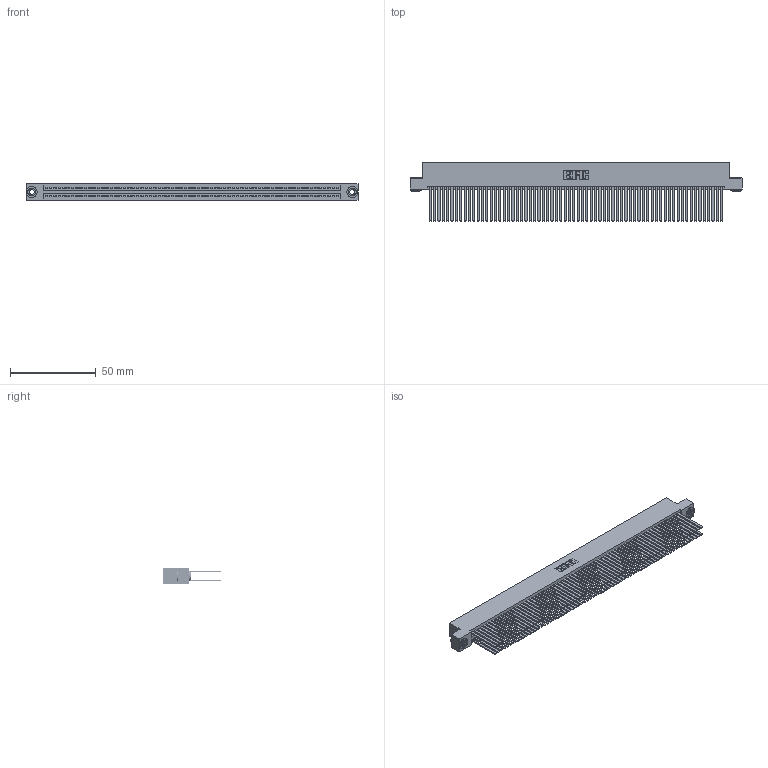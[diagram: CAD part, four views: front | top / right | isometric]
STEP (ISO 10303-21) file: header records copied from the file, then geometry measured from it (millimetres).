
FILE_DESCRIPTION (( 'STEP AP203' ), '1' );
FILE_NAME ('345-136-544-203.STEP', '2019-11-08T09:29:39', ( '' ), ( '' ), 'SwSTEP 2.0', 'SolidWorks 2016', '' );
FILE_SCHEMA (( 'CONFIG_CONTROL_DESIGN' ));
Length unit declared in the file: inch
Products named in the file (4): 345-250-002_345-250-002-102; 345-292-001_345-293-144; 345 Part_Flush Mounting Lugs - 0.156 Dia-TH; 345-136-544-203
Assembly tree (139 placements, depth 2):
  345-136-544-203
    345 Part_Flush Mounting Lugs - 0.156 Dia-TH
    345-292-001_345-293-144  x136
    345-250-002_345-250-002-102  x2
Bounding box: 193.93 x 33.96 x 9.4 mm (x, y, z)
Volume: 21005.7 mm3; surface area: 37346.1 mm2
Topology: 139 solids, 139 shells, 6148 faces, 18233 edges, 11970 vertices
Faces by surface type: plane 4034, cylinder 2106, cone 8
Entity records: 50320 total; most frequent: CARTESIAN_POINT 8383, ORIENTED_EDGE 8310, DIRECTION 7389, EDGE_CURVE 4155, LINE 3731, VECTOR 3731, VERTEX_POINT 2766, AXIS2_PLACEMENT_3D 1829
